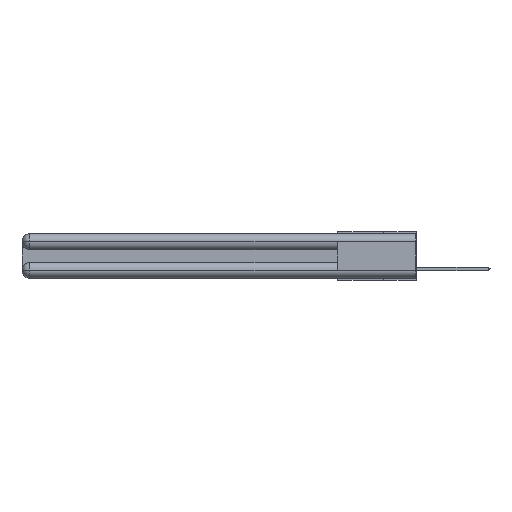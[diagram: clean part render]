
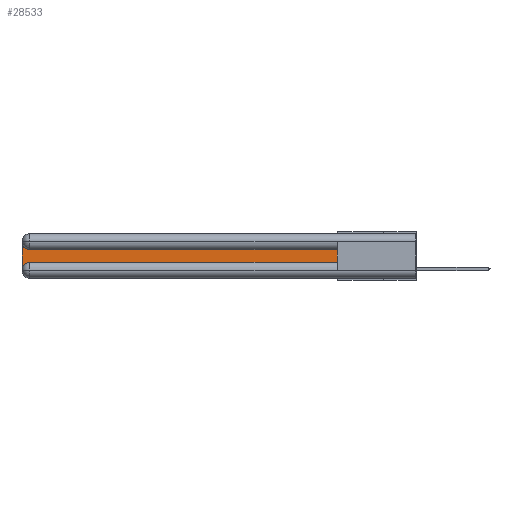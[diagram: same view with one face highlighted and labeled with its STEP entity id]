
A CAD part, left-side view. The second image highlights one B-rep face of the part: STEP entity #28533.
In plain terms, the highlighted planar face has unit normal (-1, 0, 0).
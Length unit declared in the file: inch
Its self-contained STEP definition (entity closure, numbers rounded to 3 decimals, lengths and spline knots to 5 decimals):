
#1077 = EDGE_CURVE ( 'NONE', #7168, #9656, #5502, .T. ) ;
#1195 = LINE ( 'NONE', #21608, #11616 ) ;
#2004 = FACE_OUTER_BOUND ( 'NONE', #24278, .T. ) ;
#2341 = EDGE_CURVE ( 'NONE', #18081, #29962, #9474, .T. ) ;
#3267 = LINE ( 'NONE', #15799, #27807 ) ;
#3752 = EDGE_CURVE ( 'NONE', #8470, #24313, #28645, .T. ) ;
#4913 = EDGE_CURVE ( 'NONE', #29962, #7168, #3267, .T. ) ;
#5438 = AXIS2_PLACEMENT_3D ( 'NONE', #13109, #25067, #29849 ) ;
#5502 = LINE ( 'NONE', #28005, #11890 ) ;
#5854 = DIRECTION ( 'NONE',  ( 0., 0., -1. ) ) ;
#6324 = ORIENTED_EDGE ( 'NONE', *, *, #4913, .T. ) ;
#6578 = DIRECTION ( 'NONE',  ( 1., 0., 0. ) ) ;
#7168 = VERTEX_POINT ( 'NONE', #24796 ) ;
#8025 = CARTESIAN_POINT ( 'NONE',  ( 0.075, 3., -0.2775 ) ) ;
#8470 = VERTEX_POINT ( 'NONE', #28910 ) ;
#8656 = ORIENTED_EDGE ( 'NONE', *, *, #18009, .T. ) ;
#8964 = DIRECTION ( 'NONE',  ( 0., 0., -1. ) ) ;
#9474 = CIRCLE ( 'NONE', #16746, 0.06 ) ;
#9656 = VERTEX_POINT ( 'NONE', #18351 ) ;
#10238 = EDGE_CURVE ( 'NONE', #9656, #8470, #17208, .T. ) ;
#10752 = DIRECTION ( 'NONE',  ( 0., 1., 0. ) ) ;
#11026 = DIRECTION ( 'NONE',  ( 0., -1., 0. ) ) ;
#11616 = VECTOR ( 'NONE', #28878, 39.37008 ) ;
#11890 = VECTOR ( 'NONE', #13765, 39.37008 ) ;
#13023 = CARTESIAN_POINT ( 'NONE',  ( 0.075, 0.6, -0.1225 ) ) ;
#13109 = CARTESIAN_POINT ( 'NONE',  ( 0.075, 2.94, -0.0625 ) ) ;
#13321 = DIRECTION ( 'NONE',  ( 1., 0., 0. ) ) ;
#13765 = DIRECTION ( 'NONE',  ( 0., 0., 1. ) ) ;
#14423 = CARTESIAN_POINT ( 'NONE',  ( 0.075, 2.94, -0.2175 ) ) ;
#15145 = AXIS2_PLACEMENT_3D ( 'NONE', #18279, #6578, #8964 ) ;
#15799 = CARTESIAN_POINT ( 'NONE',  ( 0.075, 0.6, -0.2175 ) ) ;
#16746 = AXIS2_PLACEMENT_3D ( 'NONE', #22560, #13321, #5854 ) ;
#17208 = LINE ( 'NONE', #13023, #20187 ) ;
#18009 = EDGE_CURVE ( 'NONE', #24313, #18081, #1195, .T. ) ;
#18081 = VERTEX_POINT ( 'NONE', #8025 ) ;
#18279 = CARTESIAN_POINT ( 'NONE',  ( 0.075, 3., -0.1225 ) ) ;
#18351 = CARTESIAN_POINT ( 'NONE',  ( 0.075, 0.6, -0.1225 ) ) ;
#18458 = CARTESIAN_POINT ( 'NONE',  ( 0.075, 3., -0.0625 ) ) ;
#20187 = VECTOR ( 'NONE', #10752, 39.37008 ) ;
#21329 = ORIENTED_EDGE ( 'NONE', *, *, #1077, .T. ) ;
#21529 = ORIENTED_EDGE ( 'NONE', *, *, #2341, .T. ) ;
#21608 = CARTESIAN_POINT ( 'NONE',  ( 0.075, 3., -0.2175 ) ) ;
#22560 = CARTESIAN_POINT ( 'NONE',  ( 0.075, 2.94, -0.2775 ) ) ;
#23178 = PLANE ( 'NONE',  #15145 ) ;
#24241 = ORIENTED_EDGE ( 'NONE', *, *, #10238, .T. ) ;
#24278 = EDGE_LOOP ( 'NONE', ( #24241, #25918, #8656, #21529, #6324, #21329 ) ) ;
#24313 = VERTEX_POINT ( 'NONE', #18458 ) ;
#24796 = CARTESIAN_POINT ( 'NONE',  ( 0.075, 0.6, -0.2175 ) ) ;
#25067 = DIRECTION ( 'NONE',  ( 1., 0., 0. ) ) ;
#25918 = ORIENTED_EDGE ( 'NONE', *, *, #3752, .T. ) ;
#27807 = VECTOR ( 'NONE', #11026, 39.37008 ) ;
#28005 = CARTESIAN_POINT ( 'NONE',  ( 0.075, 0.6, -0.2175 ) ) ;
#28533 = ADVANCED_FACE ( 'NONE', ( #2004 ), #23178, .F. ) ;
#28645 = CIRCLE ( 'NONE', #5438, 0.06 ) ;
#28878 = DIRECTION ( 'NONE',  ( 0., 0., -1. ) ) ;
#28910 = CARTESIAN_POINT ( 'NONE',  ( 0.075, 2.94, -0.1225 ) ) ;
#29849 = DIRECTION ( 'NONE',  ( 0., 0., -1. ) ) ;
#29962 = VERTEX_POINT ( 'NONE', #14423 ) ;
